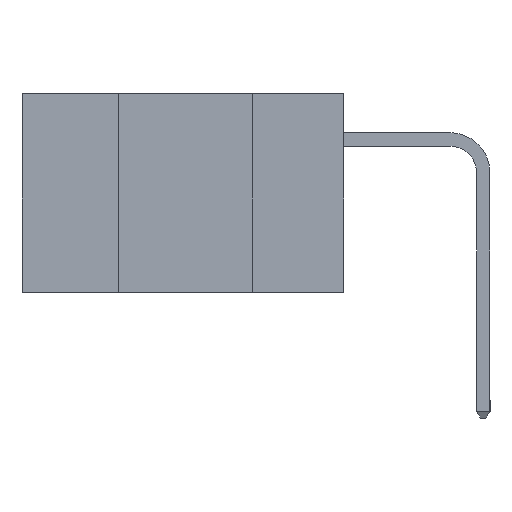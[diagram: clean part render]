
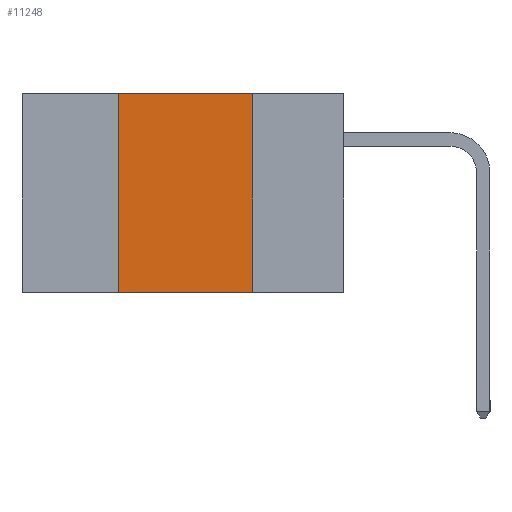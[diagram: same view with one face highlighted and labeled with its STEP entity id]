
A CAD part, left-side view. The second image highlights one B-rep face of the part: STEP entity #11248.
In plain terms, the highlighted planar face has unit normal (-1, 0, 0).
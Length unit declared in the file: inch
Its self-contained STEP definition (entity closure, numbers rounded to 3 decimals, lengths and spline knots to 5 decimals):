
#656 = CARTESIAN_POINT ( 'NONE',  ( 0., 0.6, 0. ) ) ;
#2443 = CARTESIAN_POINT ( 'NONE',  ( 0., 0.17, -0.37 ) ) ;
#2467 = EDGE_CURVE ( 'NONE', #10168, #14991, #21550, .T. ) ;
#2524 = LINE ( 'NONE', #3511, #7301 ) ;
#3511 = CARTESIAN_POINT ( 'NONE',  ( 0., 0.6, -0.37 ) ) ;
#3562 = CARTESIAN_POINT ( 'NONE',  ( 0., 0.17, 0. ) ) ;
#5923 = AXIS2_PLACEMENT_3D ( 'NONE', #656, #6800, #20984 ) ;
#6800 = DIRECTION ( 'NONE',  ( 1., 0., 0. ) ) ;
#7010 = CARTESIAN_POINT ( 'NONE',  ( 0., 0.42, -0.37 ) ) ;
#7264 = VERTEX_POINT ( 'NONE', #10694 ) ;
#7301 = VECTOR ( 'NONE', #25627, 39.37008 ) ;
#9178 = ORIENTED_EDGE ( 'NONE', *, *, #15313, .T. ) ;
#9845 = CARTESIAN_POINT ( 'NONE',  ( 0., 0.6, 0. ) ) ;
#10168 = VERTEX_POINT ( 'NONE', #3562 ) ;
#10694 = CARTESIAN_POINT ( 'NONE',  ( 0., 0.42, -0.37 ) ) ;
#11248 = ADVANCED_FACE ( 'NONE', ( #17366 ), #18950, .F. ) ;
#13151 = DIRECTION ( 'NONE',  ( 0., 0., 1. ) ) ;
#14055 = VERTEX_POINT ( 'NONE', #23642 ) ;
#14879 = CARTESIAN_POINT ( 'NONE',  ( 0., 0.17, -0.37 ) ) ;
#14973 = DIRECTION ( 'NONE',  ( 0., 0., -1. ) ) ;
#14991 = VERTEX_POINT ( 'NONE', #2443 ) ;
#15313 = EDGE_CURVE ( 'NONE', #7264, #14991, #2524, .T. ) ;
#16886 = EDGE_LOOP ( 'NONE', ( #18089, #20949, #21796, #9178 ) ) ;
#17366 = FACE_OUTER_BOUND ( 'NONE', #16886, .T. ) ;
#18089 = ORIENTED_EDGE ( 'NONE', *, *, #2467, .F. ) ;
#18950 = PLANE ( 'NONE',  #5923 ) ;
#19946 = VECTOR ( 'NONE', #13151, 39.37008 ) ;
#20033 = VECTOR ( 'NONE', #25847, 39.37008 ) ;
#20656 = EDGE_CURVE ( 'NONE', #7264, #14055, #25828, .T. ) ;
#20910 = VECTOR ( 'NONE', #14973, 39.37008 ) ;
#20949 = ORIENTED_EDGE ( 'NONE', *, *, #24649, .F. ) ;
#20984 = DIRECTION ( 'NONE',  ( 0., 0., -1. ) ) ;
#21550 = LINE ( 'NONE', #14879, #20910 ) ;
#21796 = ORIENTED_EDGE ( 'NONE', *, *, #20656, .F. ) ;
#23642 = CARTESIAN_POINT ( 'NONE',  ( 0., 0.42, 0. ) ) ;
#24649 = EDGE_CURVE ( 'NONE', #14055, #10168, #25906, .T. ) ;
#25627 = DIRECTION ( 'NONE',  ( 0., -1., 0. ) ) ;
#25828 = LINE ( 'NONE', #7010, #19946 ) ;
#25847 = DIRECTION ( 'NONE',  ( 0., -1., 0. ) ) ;
#25906 = LINE ( 'NONE', #9845, #20033 ) ;
